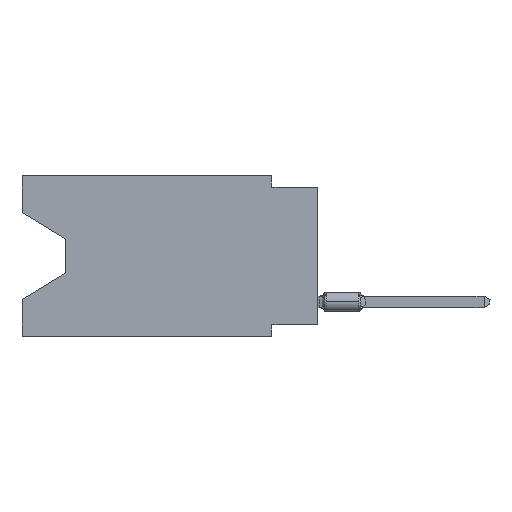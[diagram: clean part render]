
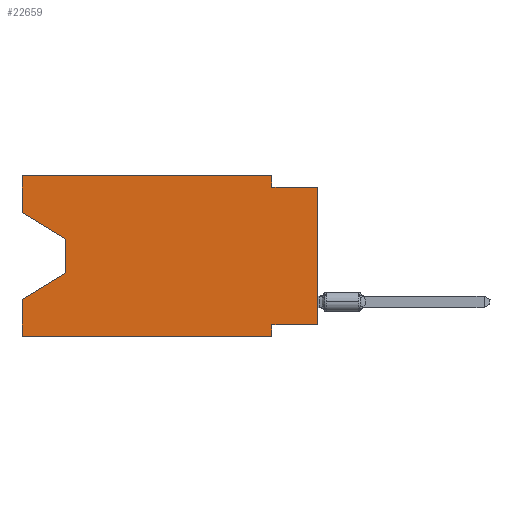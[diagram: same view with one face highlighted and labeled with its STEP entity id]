
A CAD part, left-side view. The second image highlights one B-rep face of the part: STEP entity #22659.
In plain terms, the highlighted planar face has unit normal (-1, 0, 0).
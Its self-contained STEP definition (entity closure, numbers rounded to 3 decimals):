
#102 = CARTESIAN_POINT ( 'NONE',  ( 0., 0., -8.255 ) ) ;
#157 = DIRECTION ( 'NONE',  ( 0., -1., 0. ) ) ;
#963 = EDGE_CURVE ( 'NONE', #13338, #12150, #12760, .T. ) ;
#1498 = EDGE_CURVE ( 'NONE', #15868, #30977, #32891, .T. ) ;
#1801 = LINE ( 'NONE', #11832, #21601 ) ;
#2013 = EDGE_CURVE ( 'NONE', #13338, #8145, #31005, .T. ) ;
#2704 = VECTOR ( 'NONE', #27894, 1000. ) ;
#2819 = VECTOR ( 'NONE', #23043, 1000. ) ;
#3051 = VERTEX_POINT ( 'NONE', #14990 ) ;
#3572 = CARTESIAN_POINT ( 'NONE',  ( 0., 16.383, 0. ) ) ;
#3798 = EDGE_CURVE ( 'NONE', #8145, #30591, #14855, .T. ) ;
#3830 = ORIENTED_EDGE ( 'NONE', *, *, #27062, .T. ) ;
#4445 = VERTEX_POINT ( 'NONE', #6886 ) ;
#5088 = VECTOR ( 'NONE', #29984, 1000. ) ;
#5276 = VERTEX_POINT ( 'NONE', #15266 ) ;
#6576 = LINE ( 'NONE', #16774, #31185 ) ;
#6886 = CARTESIAN_POINT ( 'NONE',  ( 0., 13.97, -3.505 ) ) ;
#7429 = EDGE_CURVE ( 'NONE', #5276, #30591, #30140, .T. ) ;
#7465 = ORIENTED_EDGE ( 'NONE', *, *, #2013, .F. ) ;
#7497 = VECTOR ( 'NONE', #28301, 1000. ) ;
#8097 = CARTESIAN_POINT ( 'NONE',  ( 0., 13.97, -5.385 ) ) ;
#8145 = VERTEX_POINT ( 'NONE', #26735 ) ;
#8775 = CARTESIAN_POINT ( 'NONE',  ( 0., 16.383, 0. ) ) ;
#9094 = ORIENTED_EDGE ( 'NONE', *, *, #11677, .T. ) ;
#9918 = LINE ( 'NONE', #12091, #5088 ) ;
#10084 = CARTESIAN_POINT ( 'NONE',  ( 0., 0., -8.255 ) ) ;
#10390 = VERTEX_POINT ( 'NONE', #24750 ) ;
#10503 = ORIENTED_EDGE ( 'NONE', *, *, #7429, .T. ) ;
#10565 = CARTESIAN_POINT ( 'NONE',  ( 0., 16.383, -8.89 ) ) ;
#11677 = EDGE_CURVE ( 'NONE', #3051, #4445, #6576, .T. ) ;
#11832 = CARTESIAN_POINT ( 'NONE',  ( 0., 13.97, -3.505 ) ) ;
#12001 = ORIENTED_EDGE ( 'NONE', *, *, #3798, .F. ) ;
#12047 = CARTESIAN_POINT ( 'NONE',  ( 0., 0., -0.635 ) ) ;
#12091 = CARTESIAN_POINT ( 'NONE',  ( 0., 13.97, -5.385 ) ) ;
#12150 = VERTEX_POINT ( 'NONE', #12047 ) ;
#12760 = LINE ( 'NONE', #13251, #7497 ) ;
#13251 = CARTESIAN_POINT ( 'NONE',  ( 0., 0., 0. ) ) ;
#13338 = VERTEX_POINT ( 'NONE', #10084 ) ;
#14050 = EDGE_CURVE ( 'NONE', #18062, #30928, #9918, .T. ) ;
#14549 = CARTESIAN_POINT ( 'NONE',  ( 0., 2.54, 0. ) ) ;
#14855 = LINE ( 'NONE', #19886, #2819 ) ;
#14912 = VECTOR ( 'NONE', #157, 1000. ) ;
#14990 = CARTESIAN_POINT ( 'NONE',  ( 0., 16.383, -2.038 ) ) ;
#15266 = CARTESIAN_POINT ( 'NONE',  ( 0., 16.383, -8.89 ) ) ;
#15868 = VERTEX_POINT ( 'NONE', #14549 ) ;
#16086 = VECTOR ( 'NONE', #18317, 1000. ) ;
#16198 = CARTESIAN_POINT ( 'NONE',  ( 0., 2.54, -0.635 ) ) ;
#16269 = ORIENTED_EDGE ( 'NONE', *, *, #22650, .F. ) ;
#16774 = CARTESIAN_POINT ( 'NONE',  ( 0., 16.383, -2.038 ) ) ;
#17036 = LINE ( 'NONE', #32559, #31277 ) ;
#17223 = ORIENTED_EDGE ( 'NONE', *, *, #963, .T. ) ;
#17706 = CARTESIAN_POINT ( 'NONE',  ( 0., 2.54, 0. ) ) ;
#17749 = ORIENTED_EDGE ( 'NONE', *, *, #32949, .F. ) ;
#18062 = VERTEX_POINT ( 'NONE', #8097 ) ;
#18240 = EDGE_CURVE ( 'NONE', #30977, #12150, #25237, .T. ) ;
#18317 = DIRECTION ( 'NONE',  ( 0., 1., 0. ) ) ;
#18893 = ORIENTED_EDGE ( 'NONE', *, *, #1498, .F. ) ;
#18963 = LINE ( 'NONE', #29148, #29309 ) ;
#18972 = DIRECTION ( 'NONE',  ( 1., 0., 0. ) ) ;
#19886 = CARTESIAN_POINT ( 'NONE',  ( 0., 2.54, -8.89 ) ) ;
#21380 = CARTESIAN_POINT ( 'NONE',  ( 0., 16.383, -6.852 ) ) ;
#21478 = FACE_OUTER_BOUND ( 'NONE', #29858, .T. ) ;
#21601 = VECTOR ( 'NONE', #24871, 1000. ) ;
#22650 = EDGE_CURVE ( 'NONE', #3051, #10390, #26489, .T. ) ;
#22659 = ADVANCED_FACE ( 'NONE', ( #21478 ), #31650, .F. ) ;
#23043 = DIRECTION ( 'NONE',  ( 0., 0., -1. ) ) ;
#23057 = CARTESIAN_POINT ( 'NONE',  ( 0., 0., -0.635 ) ) ;
#23983 = DIRECTION ( 'NONE',  ( 0., 0., 1. ) ) ;
#24750 = CARTESIAN_POINT ( 'NONE',  ( 0., 16.383, 0. ) ) ;
#24871 = DIRECTION ( 'NONE',  ( 0., 0., -1. ) ) ;
#24900 = ORIENTED_EDGE ( 'NONE', *, *, #29971, .F. ) ;
#25219 = DIRECTION ( 'NONE',  ( 0., 0., 1. ) ) ;
#25237 = LINE ( 'NONE', #23057, #14912 ) ;
#25742 = ORIENTED_EDGE ( 'NONE', *, *, #14050, .T. ) ;
#26489 = LINE ( 'NONE', #3572, #27884 ) ;
#26735 = CARTESIAN_POINT ( 'NONE',  ( 0., 2.54, -8.255 ) ) ;
#27062 = EDGE_CURVE ( 'NONE', #4445, #18062, #1801, .T. ) ;
#27144 = DIRECTION ( 'NONE',  ( 0., -1., 0. ) ) ;
#27884 = VECTOR ( 'NONE', #23983, 1000. ) ;
#27894 = DIRECTION ( 'NONE',  ( 0., 0., -1. ) ) ;
#28301 = DIRECTION ( 'NONE',  ( 0., 0., 1. ) ) ;
#29148 = CARTESIAN_POINT ( 'NONE',  ( 0., 16.383, 0. ) ) ;
#29157 = DIRECTION ( 'NONE',  ( 0., 0., -1. ) ) ;
#29300 = DIRECTION ( 'NONE',  ( 0., -0.855, -0.519 ) ) ;
#29309 = VECTOR ( 'NONE', #27144, 1000. ) ;
#29744 = ORIENTED_EDGE ( 'NONE', *, *, #18240, .F. ) ;
#29858 = EDGE_LOOP ( 'NONE', ( #9094, #3830, #25742, #24900, #10503, #12001, #7465, #17223, #29744, #18893, #17749, #16269 ) ) ;
#29932 = CARTESIAN_POINT ( 'NONE',  ( 0., 2.54, -8.89 ) ) ;
#29971 = EDGE_CURVE ( 'NONE', #5276, #30928, #17036, .T. ) ;
#29984 = DIRECTION ( 'NONE',  ( 0., 0.855, -0.519 ) ) ;
#30140 = LINE ( 'NONE', #10565, #31362 ) ;
#30294 = DIRECTION ( 'NONE',  ( 0., -1., 0. ) ) ;
#30591 = VERTEX_POINT ( 'NONE', #29932 ) ;
#30928 = VERTEX_POINT ( 'NONE', #21380 ) ;
#30977 = VERTEX_POINT ( 'NONE', #16198 ) ;
#31005 = LINE ( 'NONE', #102, #16086 ) ;
#31185 = VECTOR ( 'NONE', #29300, 1000. ) ;
#31277 = VECTOR ( 'NONE', #25219, 1000. ) ;
#31362 = VECTOR ( 'NONE', #30294, 1000. ) ;
#31650 = PLANE ( 'NONE',  #32143 ) ;
#32143 = AXIS2_PLACEMENT_3D ( 'NONE', #8775, #18972, #29157 ) ;
#32559 = CARTESIAN_POINT ( 'NONE',  ( 0., 16.383, 0. ) ) ;
#32891 = LINE ( 'NONE', #17706, #2704 ) ;
#32949 = EDGE_CURVE ( 'NONE', #10390, #15868, #18963, .T. ) ;
